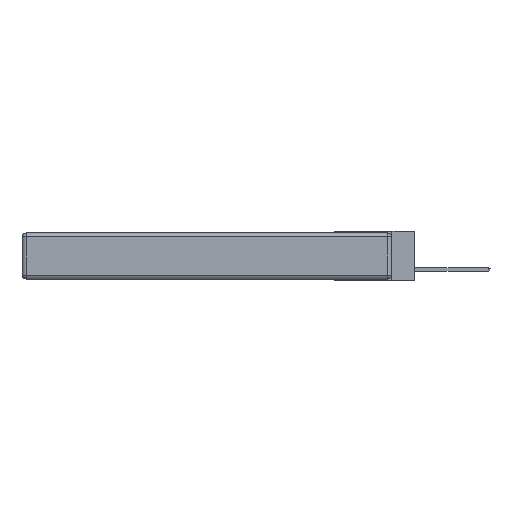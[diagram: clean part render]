
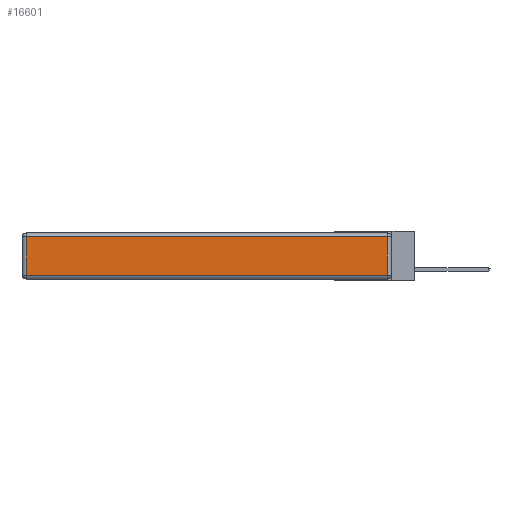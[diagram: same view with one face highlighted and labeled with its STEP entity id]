
A CAD part, left-side view. The second image highlights one B-rep face of the part: STEP entity #16601.
In plain terms, the highlighted planar face has unit normal (-1, 0, 0).
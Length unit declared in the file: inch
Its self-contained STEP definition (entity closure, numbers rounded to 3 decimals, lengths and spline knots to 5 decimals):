
#11 = LINE ( 'NONE', #9996, #15483 ) ;
#1408 = EDGE_CURVE ( 'NONE', #15429, #10407, #11, .T. ) ;
#1628 = CARTESIAN_POINT ( 'NONE',  ( 0., 0.03, -0.313 ) ) ;
#2682 = CARTESIAN_POINT ( 'NONE',  ( 0., 2.72, -0.313 ) ) ;
#6080 = CARTESIAN_POINT ( 'NONE',  ( 0., 2.72, -0.343 ) ) ;
#6489 = LINE ( 'NONE', #6080, #18514 ) ;
#7054 = EDGE_CURVE ( 'NONE', #14130, #21978, #25203, .T. ) ;
#7410 = CARTESIAN_POINT ( 'NONE',  ( 0., 0.03, -0.343 ) ) ;
#9187 = VECTOR ( 'NONE', #24563, 39.37008 ) ;
#9546 = DIRECTION ( 'NONE',  ( 0., 0., 1. ) ) ;
#9687 = DIRECTION ( 'NONE',  ( -1., 0., 0. ) ) ;
#9996 = CARTESIAN_POINT ( 'NONE',  ( 0., 2.75, -0.03 ) ) ;
#10407 = VERTEX_POINT ( 'NONE', #17698 ) ;
#11977 = DIRECTION ( 'NONE',  ( 0., 0., -1. ) ) ;
#12247 = ORIENTED_EDGE ( 'NONE', *, *, #7054, .T. ) ;
#12865 = CARTESIAN_POINT ( 'NONE',  ( 0., 0., -0.313 ) ) ;
#13484 = PLANE ( 'NONE',  #24094 ) ;
#13822 = DIRECTION ( 'NONE',  ( 0., 1., 0. ) ) ;
#14130 = VERTEX_POINT ( 'NONE', #2682 ) ;
#15026 = LINE ( 'NONE', #7410, #17810 ) ;
#15193 = DIRECTION ( 'NONE',  ( 0., 0., 1. ) ) ;
#15429 = VERTEX_POINT ( 'NONE', #20280 ) ;
#15483 = VECTOR ( 'NONE', #13822, 39.37008 ) ;
#16094 = FACE_OUTER_BOUND ( 'NONE', #21995, .T. ) ;
#16240 = ORIENTED_EDGE ( 'NONE', *, *, #1408, .T. ) ;
#16601 = ADVANCED_FACE ( 'NONE', ( #16094 ), #13484, .T. ) ;
#17048 = ORIENTED_EDGE ( 'NONE', *, *, #24814, .T. ) ;
#17698 = CARTESIAN_POINT ( 'NONE',  ( 0., 2.72, -0.03 ) ) ;
#17810 = VECTOR ( 'NONE', #9546, 39.37008 ) ;
#18012 = EDGE_CURVE ( 'NONE', #21978, #15429, #15026, .T. ) ;
#18514 = VECTOR ( 'NONE', #11977, 39.37008 ) ;
#19433 = CARTESIAN_POINT ( 'NONE',  ( 0., 0., -0.343 ) ) ;
#19629 = ORIENTED_EDGE ( 'NONE', *, *, #18012, .T. ) ;
#20280 = CARTESIAN_POINT ( 'NONE',  ( 0., 0.03, -0.03 ) ) ;
#21978 = VERTEX_POINT ( 'NONE', #1628 ) ;
#21995 = EDGE_LOOP ( 'NONE', ( #12247, #19629, #16240, #17048 ) ) ;
#24094 = AXIS2_PLACEMENT_3D ( 'NONE', #19433, #9687, #15193 ) ;
#24563 = DIRECTION ( 'NONE',  ( 0., -1., 0. ) ) ;
#24814 = EDGE_CURVE ( 'NONE', #10407, #14130, #6489, .T. ) ;
#25203 = LINE ( 'NONE', #12865, #9187 ) ;
